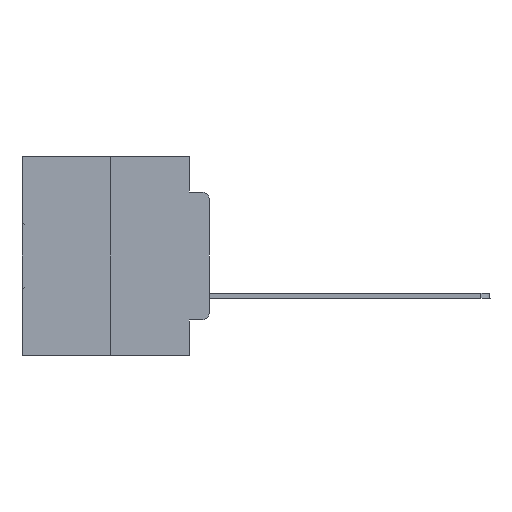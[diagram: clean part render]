
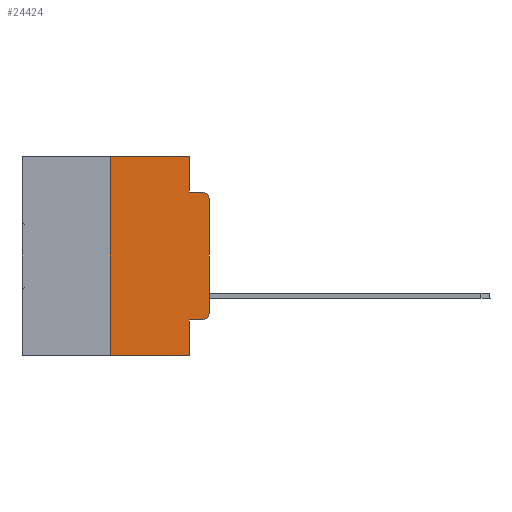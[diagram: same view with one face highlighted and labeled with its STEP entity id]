
A CAD part, left-side view. The second image highlights one B-rep face of the part: STEP entity #24424.
In plain terms, the highlighted planar face has unit normal (-1, 0, 0).
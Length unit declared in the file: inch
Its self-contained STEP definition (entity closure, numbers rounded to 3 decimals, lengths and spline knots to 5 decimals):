
#69 = CARTESIAN_POINT ( 'NONE',  ( 0., 0., -0.1085 ) ) ;
#106 = VERTEX_POINT ( 'NONE', #14725 ) ;
#310 = CARTESIAN_POINT ( 'NONE',  ( 0., 0.02, -0.3915 ) ) ;
#799 = CIRCLE ( 'NONE', #24542, 0.02 ) ;
#1559 = DIRECTION ( 'NONE',  ( 0., 0., -1. ) ) ;
#2615 = VECTOR ( 'NONE', #3014, 39.37008 ) ;
#3014 = DIRECTION ( 'NONE',  ( 0., 0., 1. ) ) ;
#3108 = CARTESIAN_POINT ( 'NONE',  ( 0., 0.25, 0. ) ) ;
#3271 = ORIENTED_EDGE ( 'NONE', *, *, #11072, .F. ) ;
#3282 = VECTOR ( 'NONE', #32745, 39.37008 ) ;
#3462 = LINE ( 'NONE', #23367, #3897 ) ;
#3654 = VERTEX_POINT ( 'NONE', #30667 ) ;
#3668 = CARTESIAN_POINT ( 'NONE',  ( 0., 0., -0.3915 ) ) ;
#3897 = VECTOR ( 'NONE', #25910, 39.37008 ) ;
#4225 = EDGE_CURVE ( 'NONE', #23162, #28801, #24155, .T. ) ;
#4437 = CARTESIAN_POINT ( 'NONE',  ( 0., 0.25, -0.5 ) ) ;
#4973 = CARTESIAN_POINT ( 'NONE',  ( 0., 0.051, -0.0885 ) ) ;
#5652 = VERTEX_POINT ( 'NONE', #4437 ) ;
#5788 = CIRCLE ( 'NONE', #18197, 0.02 ) ;
#5801 = DIRECTION ( 'NONE',  ( 0., 0., 1. ) ) ;
#5845 = LINE ( 'NONE', #27434, #31770 ) ;
#6043 = CARTESIAN_POINT ( 'NONE',  ( 0., 0.051, -0.0885 ) ) ;
#6109 = VERTEX_POINT ( 'NONE', #15819 ) ;
#6123 = DIRECTION ( 'NONE',  ( 0., 0., -1. ) ) ;
#6579 = DIRECTION ( 'NONE',  ( 0., -1., 0. ) ) ;
#6804 = EDGE_CURVE ( 'NONE', #21362, #9998, #28022, .T. ) ;
#8086 = CARTESIAN_POINT ( 'NONE',  ( 0., 0.25, 0. ) ) ;
#8161 = ORIENTED_EDGE ( 'NONE', *, *, #8431, .T. ) ;
#8431 = EDGE_CURVE ( 'NONE', #5652, #106, #15938, .T. ) ;
#8637 = EDGE_CURVE ( 'NONE', #9998, #6109, #15908, .T. ) ;
#9149 = VECTOR ( 'NONE', #30569, 39.37008 ) ;
#9180 = VECTOR ( 'NONE', #6579, 39.37008 ) ;
#9998 = VERTEX_POINT ( 'NONE', #6043 ) ;
#10176 = EDGE_LOOP ( 'NONE', ( #12864, #15993, #21562, #25968, #32006, #20502, #8161, #3271, #13206, #16355 ) ) ;
#11072 = EDGE_CURVE ( 'NONE', #21756, #106, #30305, .T. ) ;
#11679 = CARTESIAN_POINT ( 'NONE',  ( 0., 0.051, 0. ) ) ;
#11792 = FACE_OUTER_BOUND ( 'NONE', #10176, .T. ) ;
#12081 = DIRECTION ( 'NONE',  ( 0., 0., -1. ) ) ;
#12839 = LINE ( 'NONE', #3108, #25625 ) ;
#12864 = ORIENTED_EDGE ( 'NONE', *, *, #4225, .T. ) ;
#13206 = ORIENTED_EDGE ( 'NONE', *, *, #23735, .T. ) ;
#13568 = DIRECTION ( 'NONE',  ( -1., 0., 0. ) ) ;
#14725 = CARTESIAN_POINT ( 'NONE',  ( 0., 0.051, -0.5 ) ) ;
#14875 = CARTESIAN_POINT ( 'NONE',  ( 0., 0.051, 0. ) ) ;
#15819 = CARTESIAN_POINT ( 'NONE',  ( 0., 0.02, -0.0885 ) ) ;
#15908 = LINE ( 'NONE', #4973, #9149 ) ;
#15938 = LINE ( 'NONE', #16727, #9180 ) ;
#15993 = ORIENTED_EDGE ( 'NONE', *, *, #25306, .T. ) ;
#16355 = ORIENTED_EDGE ( 'NONE', *, *, #31782, .T. ) ;
#16727 = CARTESIAN_POINT ( 'NONE',  ( 0., 0.473, -0.5 ) ) ;
#16799 = DIRECTION ( 'NONE',  ( 1., 0., 0. ) ) ;
#18148 = DIRECTION ( 'NONE',  ( -1., 0., 0. ) ) ;
#18197 = AXIS2_PLACEMENT_3D ( 'NONE', #23736, #13568, #6123 ) ;
#19594 = PLANE ( 'NONE',  #29268 ) ;
#19872 = DIRECTION ( 'NONE',  ( 0., -1., 0. ) ) ;
#20502 = ORIENTED_EDGE ( 'NONE', *, *, #21166, .F. ) ;
#21166 = EDGE_CURVE ( 'NONE', #5652, #24818, #12839, .T. ) ;
#21362 = VERTEX_POINT ( 'NONE', #21369 ) ;
#21369 = CARTESIAN_POINT ( 'NONE',  ( 0., 0.051, 0. ) ) ;
#21562 = ORIENTED_EDGE ( 'NONE', *, *, #8637, .F. ) ;
#21756 = VERTEX_POINT ( 'NONE', #32201 ) ;
#23162 = VERTEX_POINT ( 'NONE', #3668 ) ;
#23368 = EDGE_CURVE ( 'NONE', #24818, #21362, #3462, .T. ) ;
#23367 = CARTESIAN_POINT ( 'NONE',  ( 0., 0.473, 0. ) ) ;
#23735 = EDGE_CURVE ( 'NONE', #21756, #3654, #5845, .T. ) ;
#23736 = CARTESIAN_POINT ( 'NONE',  ( 0., 0.02, -0.1085 ) ) ;
#24155 = LINE ( 'NONE', #25873, #2615 ) ;
#24424 = ADVANCED_FACE ( 'NONE', ( #11792 ), #19594, .F. ) ;
#24542 = AXIS2_PLACEMENT_3D ( 'NONE', #310, #18148, #25923 ) ;
#24818 = VERTEX_POINT ( 'NONE', #8086 ) ;
#25306 = EDGE_CURVE ( 'NONE', #28801, #6109, #5788, .T. ) ;
#25625 = VECTOR ( 'NONE', #5801, 39.37008 ) ;
#25873 = CARTESIAN_POINT ( 'NONE',  ( 0., 0., 0. ) ) ;
#25910 = DIRECTION ( 'NONE',  ( 0., -1., 0. ) ) ;
#25923 = DIRECTION ( 'NONE',  ( 0., 0., -1. ) ) ;
#25968 = ORIENTED_EDGE ( 'NONE', *, *, #6804, .F. ) ;
#26341 = VECTOR ( 'NONE', #1559, 39.37008 ) ;
#27369 = CARTESIAN_POINT ( 'NONE',  ( 0., 0.473, 0. ) ) ;
#27434 = CARTESIAN_POINT ( 'NONE',  ( 0., 0.051, -0.4115 ) ) ;
#28022 = LINE ( 'NONE', #14875, #3282 ) ;
#28801 = VERTEX_POINT ( 'NONE', #69 ) ;
#29268 = AXIS2_PLACEMENT_3D ( 'NONE', #27369, #16799, #12081 ) ;
#30305 = LINE ( 'NONE', #11679, #26341 ) ;
#30569 = DIRECTION ( 'NONE',  ( 0., -1., 0. ) ) ;
#30667 = CARTESIAN_POINT ( 'NONE',  ( 0., 0.02, -0.4115 ) ) ;
#31770 = VECTOR ( 'NONE', #19872, 39.37008 ) ;
#31782 = EDGE_CURVE ( 'NONE', #3654, #23162, #799, .T. ) ;
#32006 = ORIENTED_EDGE ( 'NONE', *, *, #23368, .F. ) ;
#32201 = CARTESIAN_POINT ( 'NONE',  ( 0., 0.051, -0.4115 ) ) ;
#32745 = DIRECTION ( 'NONE',  ( 0., 0., -1. ) ) ;
